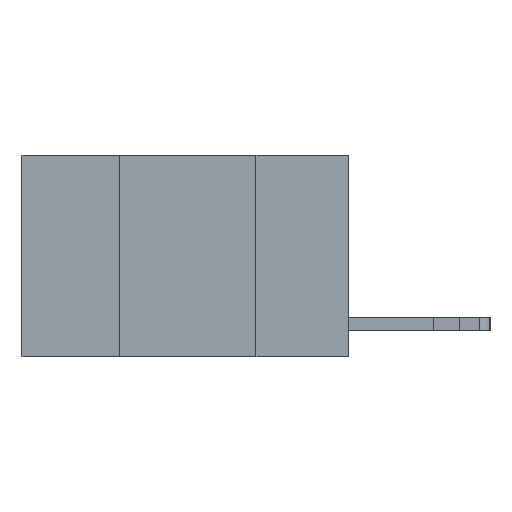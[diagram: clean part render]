
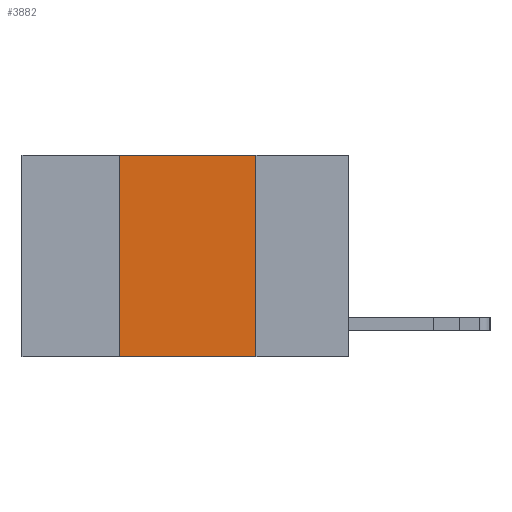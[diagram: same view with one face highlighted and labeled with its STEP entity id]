
A CAD part, left-side view. The second image highlights one B-rep face of the part: STEP entity #3882.
In plain terms, the highlighted planar face has unit normal (-1, 0, 0).
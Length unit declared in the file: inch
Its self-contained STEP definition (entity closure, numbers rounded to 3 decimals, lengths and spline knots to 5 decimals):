
#1077 = DIRECTION ( 'NONE',  ( 0., 0., -1. ) ) ;
#1182 = CARTESIAN_POINT ( 'NONE',  ( 0., 0.17, -0.37 ) ) ;
#2642 = VECTOR ( 'NONE', #16982, 39.37008 ) ;
#2887 = LINE ( 'NONE', #18128, #7473 ) ;
#3115 = VERTEX_POINT ( 'NONE', #1182 ) ;
#3162 = LINE ( 'NONE', #4990, #9495 ) ;
#3882 = ADVANCED_FACE ( 'NONE', ( #9039 ), #10646, .F. ) ;
#4699 = ORIENTED_EDGE ( 'NONE', *, *, #6626, .F. ) ;
#4990 = CARTESIAN_POINT ( 'NONE',  ( 0., 0.6, -0.37 ) ) ;
#5499 = CARTESIAN_POINT ( 'NONE',  ( 0., 0.17, 0. ) ) ;
#5639 = VECTOR ( 'NONE', #1077, 39.37008 ) ;
#5709 = LINE ( 'NONE', #18408, #2642 ) ;
#6493 = VERTEX_POINT ( 'NONE', #14894 ) ;
#6626 = EDGE_CURVE ( 'NONE', #15789, #3115, #9623, .T. ) ;
#6830 = EDGE_CURVE ( 'NONE', #6493, #3115, #3162, .T. ) ;
#7303 = ORIENTED_EDGE ( 'NONE', *, *, #7574, .F. ) ;
#7473 = VECTOR ( 'NONE', #14329, 39.37008 ) ;
#7574 = EDGE_CURVE ( 'NONE', #15375, #15789, #5709, .T. ) ;
#7636 = DIRECTION ( 'NONE',  ( 0., 0., -1. ) ) ;
#9039 = FACE_OUTER_BOUND ( 'NONE', #17521, .T. ) ;
#9262 = ORIENTED_EDGE ( 'NONE', *, *, #14269, .F. ) ;
#9495 = VECTOR ( 'NONE', #11711, 39.37008 ) ;
#9623 = LINE ( 'NONE', #5499, #5639 ) ;
#10646 = PLANE ( 'NONE',  #11845 ) ;
#11309 = CARTESIAN_POINT ( 'NONE',  ( 0., 0.17, 0. ) ) ;
#11711 = DIRECTION ( 'NONE',  ( 0., -1., 0. ) ) ;
#11845 = AXIS2_PLACEMENT_3D ( 'NONE', #11888, #16366, #7636 ) ;
#11888 = CARTESIAN_POINT ( 'NONE',  ( 0., 0.6, 0. ) ) ;
#14269 = EDGE_CURVE ( 'NONE', #6493, #15375, #2887, .T. ) ;
#14329 = DIRECTION ( 'NONE',  ( 0., 0., 1. ) ) ;
#14651 = ORIENTED_EDGE ( 'NONE', *, *, #6830, .T. ) ;
#14894 = CARTESIAN_POINT ( 'NONE',  ( 0., 0.42, -0.37 ) ) ;
#15375 = VERTEX_POINT ( 'NONE', #18375 ) ;
#15789 = VERTEX_POINT ( 'NONE', #11309 ) ;
#16366 = DIRECTION ( 'NONE',  ( 1., 0., 0. ) ) ;
#16982 = DIRECTION ( 'NONE',  ( 0., -1., 0. ) ) ;
#17521 = EDGE_LOOP ( 'NONE', ( #4699, #7303, #9262, #14651 ) ) ;
#18128 = CARTESIAN_POINT ( 'NONE',  ( 0., 0.42, 0. ) ) ;
#18375 = CARTESIAN_POINT ( 'NONE',  ( 0., 0.42, 0. ) ) ;
#18408 = CARTESIAN_POINT ( 'NONE',  ( 0., 0.6, 0. ) ) ;
